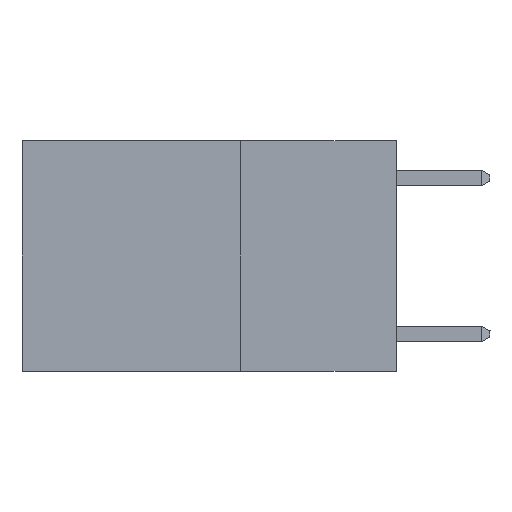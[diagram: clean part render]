
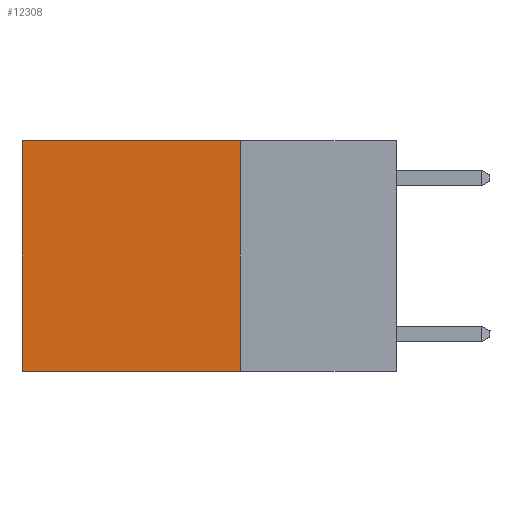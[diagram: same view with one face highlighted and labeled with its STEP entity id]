
A CAD part, left-side view. The second image highlights one B-rep face of the part: STEP entity #12308.
In plain terms, the highlighted planar face has unit normal (-1, 0, 0).
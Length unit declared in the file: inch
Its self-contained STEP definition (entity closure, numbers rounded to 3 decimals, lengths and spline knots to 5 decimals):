
#567 = DIRECTION ( 'NONE',  ( 0., 1., 0. ) ) ;
#1084 = EDGE_CURVE ( 'NONE', #6003, #2355, #7547, .T. ) ;
#2258 = DIRECTION ( 'NONE',  ( 1., 0., 0. ) ) ;
#2355 = VERTEX_POINT ( 'NONE', #6373 ) ;
#2705 = EDGE_CURVE ( 'NONE', #12370, #14540, #14662, .T. ) ;
#2837 = ORIENTED_EDGE ( 'NONE', *, *, #5867, .T. ) ;
#2874 = DIRECTION ( 'NONE',  ( 0., 1., 0. ) ) ;
#3294 = CARTESIAN_POINT ( 'NONE',  ( 0.2625, 0.25, -0.37 ) ) ;
#3692 = VECTOR ( 'NONE', #13041, 39.37008 ) ;
#3891 = CARTESIAN_POINT ( 'NONE',  ( 0.2625, 0.25, -0.37 ) ) ;
#3968 = VECTOR ( 'NONE', #2874, 39.37008 ) ;
#4014 = ORIENTED_EDGE ( 'NONE', *, *, #2705, .F. ) ;
#4359 = DIRECTION ( 'NONE',  ( 0., 0., -1. ) ) ;
#4491 = ORIENTED_EDGE ( 'NONE', *, *, #4776, .F. ) ;
#4776 = EDGE_CURVE ( 'NONE', #6003, #12370, #7266, .T. ) ;
#4930 = CARTESIAN_POINT ( 'NONE',  ( 0.2625, 0.6, -0.37 ) ) ;
#5357 = ORIENTED_EDGE ( 'NONE', *, *, #1084, .T. ) ;
#5867 = EDGE_CURVE ( 'NONE', #2355, #14540, #12671, .T. ) ;
#6003 = VERTEX_POINT ( 'NONE', #13999 ) ;
#6324 = CARTESIAN_POINT ( 'NONE',  ( 0.2625, 0.25, 0. ) ) ;
#6373 = CARTESIAN_POINT ( 'NONE',  ( 0.2625, 0.6, 0. ) ) ;
#6486 = EDGE_LOOP ( 'NONE', ( #2837, #4014, #4491, #5357 ) ) ;
#7022 = CARTESIAN_POINT ( 'NONE',  ( 0.2625, 0.6, 0. ) ) ;
#7266 = LINE ( 'NONE', #12982, #3692 ) ;
#7547 = LINE ( 'NONE', #12263, #3968 ) ;
#7601 = PLANE ( 'NONE',  #13727 ) ;
#9075 = VECTOR ( 'NONE', #4359, 39.37008 ) ;
#11708 = DIRECTION ( 'NONE',  ( 0., 0., -1. ) ) ;
#12263 = CARTESIAN_POINT ( 'NONE',  ( 0.2625, 0.25, 0. ) ) ;
#12308 = ADVANCED_FACE ( 'NONE', ( #17108 ), #7601, .F. ) ;
#12370 = VERTEX_POINT ( 'NONE', #3891 ) ;
#12671 = LINE ( 'NONE', #7022, #9075 ) ;
#12982 = CARTESIAN_POINT ( 'NONE',  ( 0.2625, 0.25, 0. ) ) ;
#13041 = DIRECTION ( 'NONE',  ( 0., 0., -1. ) ) ;
#13727 = AXIS2_PLACEMENT_3D ( 'NONE', #6324, #2258, #11708 ) ;
#13999 = CARTESIAN_POINT ( 'NONE',  ( 0.2625, 0.25, 0. ) ) ;
#14250 = VECTOR ( 'NONE', #567, 39.37008 ) ;
#14540 = VERTEX_POINT ( 'NONE', #4930 ) ;
#14662 = LINE ( 'NONE', #3294, #14250 ) ;
#17108 = FACE_OUTER_BOUND ( 'NONE', #6486, .T. ) ;
